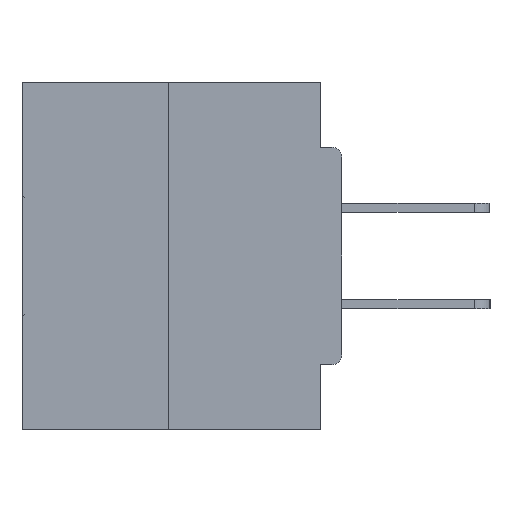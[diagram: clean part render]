
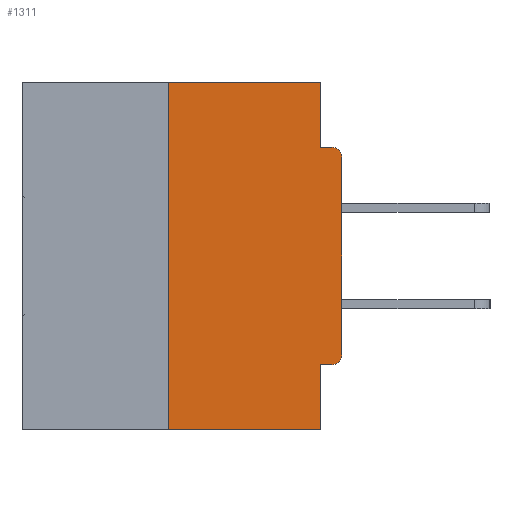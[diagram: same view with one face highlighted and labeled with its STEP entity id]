
A CAD part, left-side view. The second image highlights one B-rep face of the part: STEP entity #1311.
In plain terms, the highlighted planar face has unit normal (-1, 0, 0).
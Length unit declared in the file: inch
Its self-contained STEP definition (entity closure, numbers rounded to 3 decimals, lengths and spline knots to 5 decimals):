
#348 = VECTOR ( 'NONE', #33075, 39.37008 ) ;
#1080 = DIRECTION ( 'NONE',  ( 0., 0., -1. ) ) ;
#1311 = ADVANCED_FACE ( 'NONE', ( #30167 ), #14607, .F. ) ;
#1746 = VERTEX_POINT ( 'NONE', #31318 ) ;
#2052 = LINE ( 'NONE', #14955, #17833 ) ;
#2096 = VERTEX_POINT ( 'NONE', #22988 ) ;
#2137 = EDGE_CURVE ( 'NONE', #29826, #11274, #10852, .T. ) ;
#2482 = EDGE_CURVE ( 'NONE', #40052, #16031, #26161, .T. ) ;
#3161 = CARTESIAN_POINT ( 'NONE',  ( 0., 0., -0.4065 ) ) ;
#3185 = VECTOR ( 'NONE', #16083, 39.37008 ) ;
#3880 = DIRECTION ( 'NONE',  ( 0., -1., 0. ) ) ;
#4520 = DIRECTION ( 'NONE',  ( 0., -1., 0. ) ) ;
#4927 = CARTESIAN_POINT ( 'NONE',  ( 0., 0.015, -0.4065 ) ) ;
#5060 = DIRECTION ( 'NONE',  ( 0., 0., -1. ) ) ;
#5635 = ORIENTED_EDGE ( 'NONE', *, *, #2137, .F. ) ;
#6240 = VECTOR ( 'NONE', #3880, 39.37008 ) ;
#6812 = CARTESIAN_POINT ( 'NONE',  ( 0., 0.031, -0.0935 ) ) ;
#7405 = ORIENTED_EDGE ( 'NONE', *, *, #2482, .T. ) ;
#9058 = EDGE_LOOP ( 'NONE', ( #28731, #14800, #39231, #27091, #21179, #7405, #16769, #17537, #5635, #25730 ) ) ;
#9536 = LINE ( 'NONE', #3161, #3185 ) ;
#9837 = CARTESIAN_POINT ( 'NONE',  ( 0., 0.46, -0.5 ) ) ;
#10852 = LINE ( 'NONE', #24265, #29511 ) ;
#10969 = CARTESIAN_POINT ( 'NONE',  ( 0., 0., -0.3915 ) ) ;
#11015 = DIRECTION ( 'NONE',  ( 1., 0., 0. ) ) ;
#11176 = DIRECTION ( 'NONE',  ( 0., 0., -1. ) ) ;
#11274 = VERTEX_POINT ( 'NONE', #34105 ) ;
#11504 = CARTESIAN_POINT ( 'NONE',  ( 0., 0.031, 0. ) ) ;
#11712 = CIRCLE ( 'NONE', #23944, 0.015 ) ;
#12744 = CARTESIAN_POINT ( 'NONE',  ( 0., 0.031, -0.5 ) ) ;
#14607 = PLANE ( 'NONE',  #22851 ) ;
#14800 = ORIENTED_EDGE ( 'NONE', *, *, #20976, .F. ) ;
#14955 = CARTESIAN_POINT ( 'NONE',  ( 0., 0., 0. ) ) ;
#15519 = EDGE_CURVE ( 'NONE', #19387, #1746, #38859, .T. ) ;
#15690 = CARTESIAN_POINT ( 'NONE',  ( 0., 0., -0.1085 ) ) ;
#15791 = DIRECTION ( 'NONE',  ( 0., 0., -1. ) ) ;
#16031 = VERTEX_POINT ( 'NONE', #10969 ) ;
#16083 = DIRECTION ( 'NONE',  ( 0., 1., 0. ) ) ;
#16769 = ORIENTED_EDGE ( 'NONE', *, *, #25853, .T. ) ;
#17537 = ORIENTED_EDGE ( 'NONE', *, *, #31930, .T. ) ;
#17833 = VECTOR ( 'NONE', #40906, 39.37008 ) ;
#18754 = CARTESIAN_POINT ( 'NONE',  ( 0., 0.25, 0. ) ) ;
#18990 = LINE ( 'NONE', #31983, #41523 ) ;
#19387 = VERTEX_POINT ( 'NONE', #39806 ) ;
#19697 = VERTEX_POINT ( 'NONE', #22365 ) ;
#20674 = EDGE_CURVE ( 'NONE', #40052, #19387, #9536, .T. ) ;
#20976 = EDGE_CURVE ( 'NONE', #2096, #19697, #38298, .T. ) ;
#21179 = ORIENTED_EDGE ( 'NONE', *, *, #20674, .F. ) ;
#22365 = CARTESIAN_POINT ( 'NONE',  ( 0., 0.25, 0. ) ) ;
#22851 = AXIS2_PLACEMENT_3D ( 'NONE', #23996, #11015, #1080 ) ;
#22988 = CARTESIAN_POINT ( 'NONE',  ( 0., 0.25, -0.5 ) ) ;
#23944 = AXIS2_PLACEMENT_3D ( 'NONE', #37300, #30550, #5060 ) ;
#23996 = CARTESIAN_POINT ( 'NONE',  ( 0., 0.46, 0. ) ) ;
#24265 = CARTESIAN_POINT ( 'NONE',  ( 0., 0., -0.0935 ) ) ;
#24502 = EDGE_CURVE ( 'NONE', #2096, #1746, #32769, .T. ) ;
#25730 = ORIENTED_EDGE ( 'NONE', *, *, #28987, .F. ) ;
#25853 = EDGE_CURVE ( 'NONE', #16031, #28140, #2052, .T. ) ;
#26161 = CIRCLE ( 'NONE', #41777, 0.015 ) ;
#26901 = CARTESIAN_POINT ( 'NONE',  ( 0., 0.015, -0.3915 ) ) ;
#27091 = ORIENTED_EDGE ( 'NONE', *, *, #15519, .F. ) ;
#28140 = VERTEX_POINT ( 'NONE', #15690 ) ;
#28731 = ORIENTED_EDGE ( 'NONE', *, *, #38950, .F. ) ;
#28963 = VECTOR ( 'NONE', #41725, 39.37008 ) ;
#28987 = EDGE_CURVE ( 'NONE', #34455, #29826, #18990, .T. ) ;
#29511 = VECTOR ( 'NONE', #4520, 39.37008 ) ;
#29826 = VERTEX_POINT ( 'NONE', #6812 ) ;
#30167 = FACE_OUTER_BOUND ( 'NONE', #9058, .T. ) ;
#30536 = DIRECTION ( 'NONE',  ( -1., 0., 0. ) ) ;
#30550 = DIRECTION ( 'NONE',  ( -1., 0., 0. ) ) ;
#31318 = CARTESIAN_POINT ( 'NONE',  ( 0., 0.031, -0.5 ) ) ;
#31930 = EDGE_CURVE ( 'NONE', #28140, #11274, #11712, .T. ) ;
#31983 = CARTESIAN_POINT ( 'NONE',  ( 0., 0.031, 0. ) ) ;
#32769 = LINE ( 'NONE', #9837, #6240 ) ;
#32936 = DIRECTION ( 'NONE',  ( 0., 0., -1. ) ) ;
#33075 = DIRECTION ( 'NONE',  ( 0., -1., 0. ) ) ;
#34105 = CARTESIAN_POINT ( 'NONE',  ( 0., 0.015, -0.0935 ) ) ;
#34455 = VERTEX_POINT ( 'NONE', #11504 ) ;
#35616 = LINE ( 'NONE', #38795, #348 ) ;
#37300 = CARTESIAN_POINT ( 'NONE',  ( 0., 0.015, -0.1085 ) ) ;
#38298 = LINE ( 'NONE', #18754, #28963 ) ;
#38795 = CARTESIAN_POINT ( 'NONE',  ( 0., 0.46, 0. ) ) ;
#38859 = LINE ( 'NONE', #12744, #40144 ) ;
#38950 = EDGE_CURVE ( 'NONE', #19697, #34455, #35616, .T. ) ;
#39231 = ORIENTED_EDGE ( 'NONE', *, *, #24502, .T. ) ;
#39806 = CARTESIAN_POINT ( 'NONE',  ( 0., 0.031, -0.4065 ) ) ;
#40052 = VERTEX_POINT ( 'NONE', #4927 ) ;
#40144 = VECTOR ( 'NONE', #32936, 39.37008 ) ;
#40906 = DIRECTION ( 'NONE',  ( 0., 0., 1. ) ) ;
#41523 = VECTOR ( 'NONE', #15791, 39.37008 ) ;
#41725 = DIRECTION ( 'NONE',  ( 0., 0., 1. ) ) ;
#41777 = AXIS2_PLACEMENT_3D ( 'NONE', #26901, #30536, #11176 ) ;
